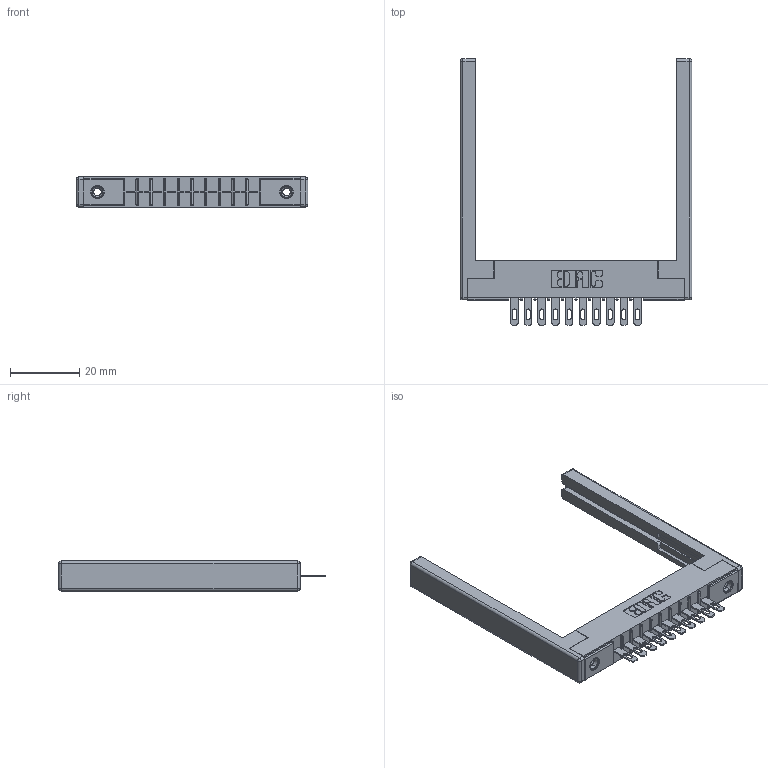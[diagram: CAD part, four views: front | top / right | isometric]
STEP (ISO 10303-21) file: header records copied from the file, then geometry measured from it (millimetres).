
FILE_DESCRIPTION (( 'STEP AP203' ), '1' );
FILE_NAME ('316-010-400-168.STEP', '2020-09-22T15:14:53', ( '' ), ( '' ), 'SwSTEP 2.0', 'SolidWorks 2020', '' );
FILE_SCHEMA (( 'CONFIG_CONTROL_DESIGN' ));
Length unit declared in the file: inch
Products named in the file (5): 306 Part_.156 Dia; 306-290-001_100; 307-220-068; 316-010-400-168; 345-250-001_345-250-001-102
Assembly tree (15 placements, depth 2):
  316-010-400-168
    306 Part_.156 Dia
    306-290-001_100  x10
    345-250-001_345-250-001-102  x2
    307-220-068  x2
Bounding box: 67.06 x 77.17 x 8.71 mm (x, y, z)
Volume: 9117.6 mm3; surface area: 10640 mm2
Topology: 15 solids, 15 shells, 1030 faces, 2856 edges, 1828 vertices
Faces by surface type: plane 656, cylinder 310, sphere 48, cone 12, torus 4
Entity records: 16394 total; most frequent: CARTESIAN_POINT 2714, DIRECTION 2693, ORIENTED_EDGE 2678, EDGE_CURVE 1339, LINE 1023, VECTOR 1023, VERTEX_POINT 856, AXIS2_PLACEMENT_3D 835
